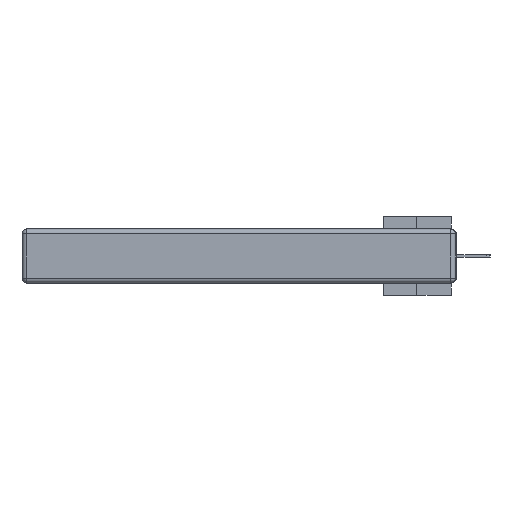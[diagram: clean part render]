
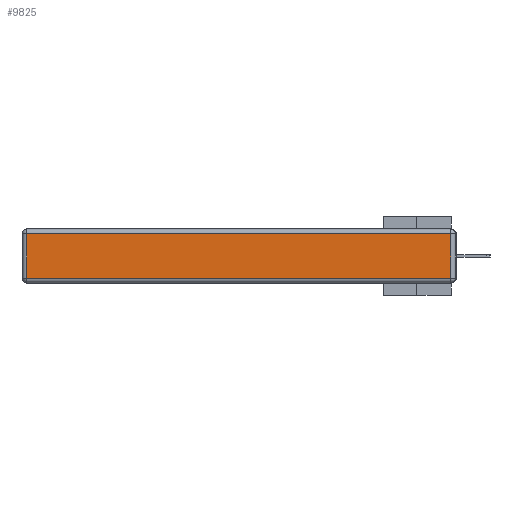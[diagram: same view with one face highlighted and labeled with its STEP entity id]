
A CAD part, left-side view. The second image highlights one B-rep face of the part: STEP entity #9825.
In plain terms, the highlighted planar face has unit normal (-1, 0, 0).
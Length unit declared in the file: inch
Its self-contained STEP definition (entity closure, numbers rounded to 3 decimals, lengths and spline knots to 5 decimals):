
#415 = LINE ( 'NONE', #3221, #35096 ) ;
#438 = DIRECTION ( 'NONE',  ( 0., 1., 0. ) ) ;
#966 = EDGE_CURVE ( 'NONE', #33594, #3484, #16779, .T. ) ;
#2008 = VECTOR ( 'NONE', #15976, 39.37008 ) ;
#2231 = CARTESIAN_POINT ( 'NONE',  ( 0., 0.03, -0.313 ) ) ;
#2936 = CARTESIAN_POINT ( 'NONE',  ( 0., 2.72, -0.03 ) ) ;
#3221 = CARTESIAN_POINT ( 'NONE',  ( 0., 2.75, -0.03 ) ) ;
#3484 = VERTEX_POINT ( 'NONE', #29629 ) ;
#3747 = CARTESIAN_POINT ( 'NONE',  ( 0., 0.03, -0.03 ) ) ;
#5243 = ORIENTED_EDGE ( 'NONE', *, *, #966, .T. ) ;
#6410 = PLANE ( 'NONE',  #15550 ) ;
#7111 = CARTESIAN_POINT ( 'NONE',  ( 0., 0., -0.313 ) ) ;
#8051 = VERTEX_POINT ( 'NONE', #2231 ) ;
#9155 = EDGE_LOOP ( 'NONE', ( #34483, #13222, #19621, #5243 ) ) ;
#9825 = ADVANCED_FACE ( 'NONE', ( #13403 ), #6410, .T. ) ;
#10977 = EDGE_CURVE ( 'NONE', #8051, #30819, #26594, .T. ) ;
#12006 = DIRECTION ( 'NONE',  ( 0., 0., 1. ) ) ;
#13222 = ORIENTED_EDGE ( 'NONE', *, *, #10977, .T. ) ;
#13403 = FACE_OUTER_BOUND ( 'NONE', #9155, .T. ) ;
#14657 = CARTESIAN_POINT ( 'NONE',  ( 0., 0., -0.343 ) ) ;
#15219 = EDGE_CURVE ( 'NONE', #30819, #33594, #415, .T. ) ;
#15491 = DIRECTION ( 'NONE',  ( 0., -1., 0. ) ) ;
#15550 = AXIS2_PLACEMENT_3D ( 'NONE', #14657, #28387, #12006 ) ;
#15976 = DIRECTION ( 'NONE',  ( 0., 0., -1. ) ) ;
#16779 = LINE ( 'NONE', #34841, #2008 ) ;
#18720 = LINE ( 'NONE', #7111, #31422 ) ;
#19621 = ORIENTED_EDGE ( 'NONE', *, *, #15219, .T. ) ;
#20157 = DIRECTION ( 'NONE',  ( 0., 0., 1. ) ) ;
#25609 = CARTESIAN_POINT ( 'NONE',  ( 0., 0.03, -0.343 ) ) ;
#26594 = LINE ( 'NONE', #25609, #32895 ) ;
#28387 = DIRECTION ( 'NONE',  ( -1., 0., 0. ) ) ;
#29629 = CARTESIAN_POINT ( 'NONE',  ( 0., 2.72, -0.313 ) ) ;
#30819 = VERTEX_POINT ( 'NONE', #3747 ) ;
#31422 = VECTOR ( 'NONE', #15491, 39.37008 ) ;
#31558 = EDGE_CURVE ( 'NONE', #3484, #8051, #18720, .T. ) ;
#32895 = VECTOR ( 'NONE', #20157, 39.37008 ) ;
#33594 = VERTEX_POINT ( 'NONE', #2936 ) ;
#34483 = ORIENTED_EDGE ( 'NONE', *, *, #31558, .T. ) ;
#34841 = CARTESIAN_POINT ( 'NONE',  ( 0., 2.72, -0.343 ) ) ;
#35096 = VECTOR ( 'NONE', #438, 39.37008 ) ;
